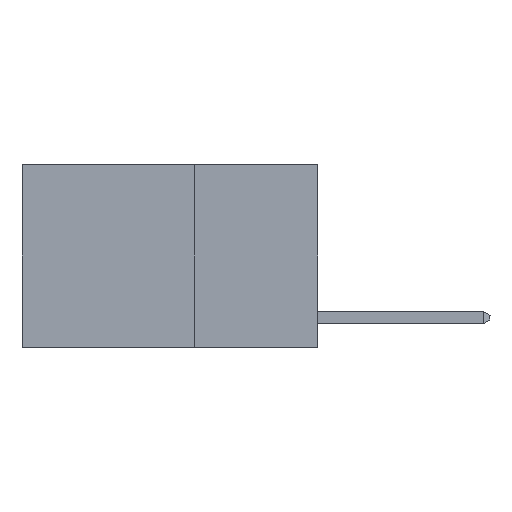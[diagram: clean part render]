
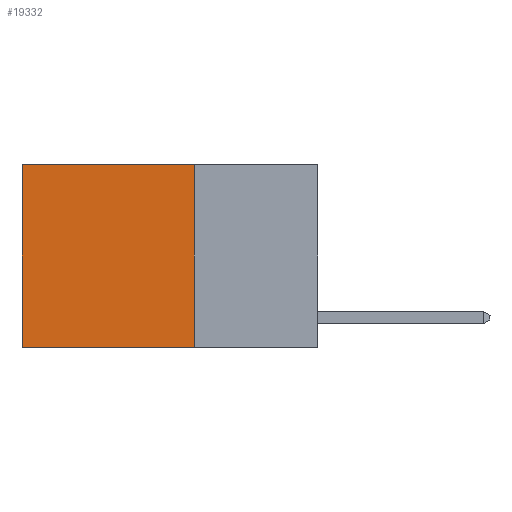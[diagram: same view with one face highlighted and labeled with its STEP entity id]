
A CAD part, left-side view. The second image highlights one B-rep face of the part: STEP entity #19332.
In plain terms, the highlighted planar face has unit normal (-1, 0, 0).
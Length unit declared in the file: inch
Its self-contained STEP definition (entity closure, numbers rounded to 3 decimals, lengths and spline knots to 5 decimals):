
#34 = LINE ( 'NONE', #3216, #15638 ) ;
#536 = VERTEX_POINT ( 'NONE', #22975 ) ;
#794 = FACE_OUTER_BOUND ( 'NONE', #5343, .T. ) ;
#1655 = CARTESIAN_POINT ( 'NONE',  ( 0.2625, 0.6, -0.37 ) ) ;
#3038 = CARTESIAN_POINT ( 'NONE',  ( 0.2625, 0.25, -0.37 ) ) ;
#3129 = EDGE_CURVE ( 'NONE', #536, #11410, #5010, .T. ) ;
#3216 = CARTESIAN_POINT ( 'NONE',  ( 0.2625, 0.6, 0. ) ) ;
#3602 = DIRECTION ( 'NONE',  ( 0., 1., 0. ) ) ;
#3756 = ORIENTED_EDGE ( 'NONE', *, *, #23317, .F. ) ;
#4218 = DIRECTION ( 'NONE',  ( 0., 1., 0. ) ) ;
#5010 = LINE ( 'NONE', #15688, #15772 ) ;
#5343 = EDGE_LOOP ( 'NONE', ( #9816, #3756, #16071, #12979 ) ) ;
#5432 = VERTEX_POINT ( 'NONE', #21500 ) ;
#6672 = VECTOR ( 'NONE', #4218, 39.37008 ) ;
#8723 = VERTEX_POINT ( 'NONE', #1655 ) ;
#8739 = EDGE_CURVE ( 'NONE', #5432, #8723, #34, .T. ) ;
#9816 = ORIENTED_EDGE ( 'NONE', *, *, #8739, .T. ) ;
#10412 = DIRECTION ( 'NONE',  ( 0., 0., -1. ) ) ;
#10549 = DIRECTION ( 'NONE',  ( 0., 0., -1. ) ) ;
#11410 = VERTEX_POINT ( 'NONE', #3038 ) ;
#12814 = CARTESIAN_POINT ( 'NONE',  ( 0.2625, 0.25, -0.37 ) ) ;
#12979 = ORIENTED_EDGE ( 'NONE', *, *, #18537, .T. ) ;
#13597 = CARTESIAN_POINT ( 'NONE',  ( 0.2625, 0.25, 0. ) ) ;
#15432 = VECTOR ( 'NONE', #3602, 39.37008 ) ;
#15638 = VECTOR ( 'NONE', #10412, 39.37008 ) ;
#15688 = CARTESIAN_POINT ( 'NONE',  ( 0.2625, 0.25, 0. ) ) ;
#15772 = VECTOR ( 'NONE', #10549, 39.37008 ) ;
#16071 = ORIENTED_EDGE ( 'NONE', *, *, #3129, .F. ) ;
#17127 = CARTESIAN_POINT ( 'NONE',  ( 0.2625, 0.25, 0. ) ) ;
#18537 = EDGE_CURVE ( 'NONE', #536, #5432, #22215, .T. ) ;
#18600 = DIRECTION ( 'NONE',  ( 0., 0., -1. ) ) ;
#18709 = DIRECTION ( 'NONE',  ( 1., 0., 0. ) ) ;
#19047 = PLANE ( 'NONE',  #19457 ) ;
#19332 = ADVANCED_FACE ( 'NONE', ( #794 ), #19047, .F. ) ;
#19457 = AXIS2_PLACEMENT_3D ( 'NONE', #13597, #18709, #18600 ) ;
#19951 = LINE ( 'NONE', #12814, #15432 ) ;
#21500 = CARTESIAN_POINT ( 'NONE',  ( 0.2625, 0.6, 0. ) ) ;
#22215 = LINE ( 'NONE', #17127, #6672 ) ;
#22975 = CARTESIAN_POINT ( 'NONE',  ( 0.2625, 0.25, 0. ) ) ;
#23317 = EDGE_CURVE ( 'NONE', #11410, #8723, #19951, .T. ) ;
